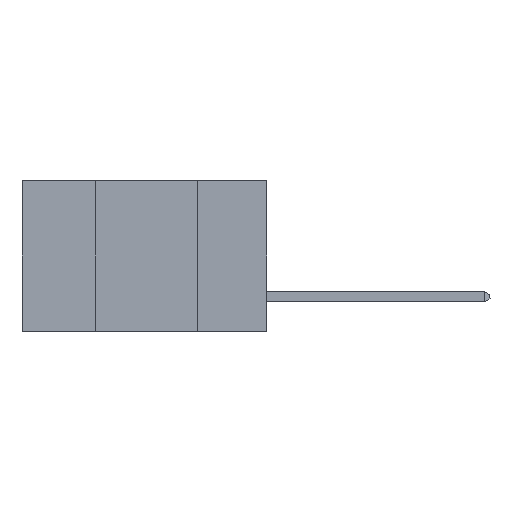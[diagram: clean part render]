
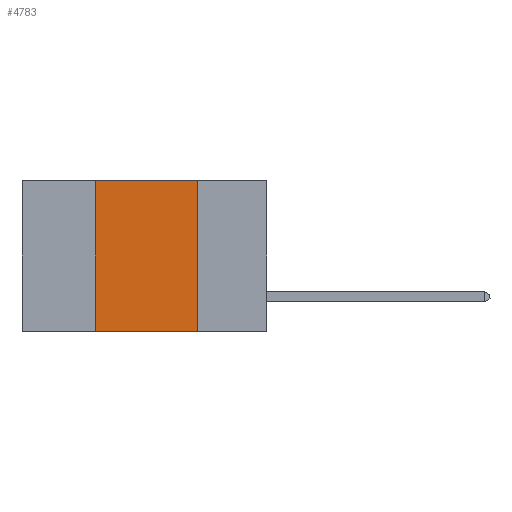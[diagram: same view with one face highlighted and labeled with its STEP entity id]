
A CAD part, left-side view. The second image highlights one B-rep face of the part: STEP entity #4783.
In plain terms, the highlighted planar face has unit normal (-1, 0, 0).
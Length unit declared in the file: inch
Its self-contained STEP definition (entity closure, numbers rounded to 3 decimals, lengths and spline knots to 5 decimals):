
#165 = EDGE_CURVE ( 'NONE', #9368, #6604, #4539, .T. ) ;
#804 = CARTESIAN_POINT ( 'NONE',  ( 0., 0.42, 0. ) ) ;
#1137 = CARTESIAN_POINT ( 'NONE',  ( 0., 0.6, 0. ) ) ;
#1305 = PLANE ( 'NONE',  #2064 ) ;
#1721 = CARTESIAN_POINT ( 'NONE',  ( 0., 0.42, -0.37 ) ) ;
#1871 = ORIENTED_EDGE ( 'NONE', *, *, #9685, .F. ) ;
#2020 = DIRECTION ( 'NONE',  ( 0., -1., 0. ) ) ;
#2064 = AXIS2_PLACEMENT_3D ( 'NONE', #1137, #6656, #10826 ) ;
#2106 = DIRECTION ( 'NONE',  ( 0., -1., 0. ) ) ;
#2413 = ORIENTED_EDGE ( 'NONE', *, *, #9881, .T. ) ;
#2480 = VERTEX_POINT ( 'NONE', #1721 ) ;
#2766 = CARTESIAN_POINT ( 'NONE',  ( 0., 0.17, -0.37 ) ) ;
#2978 = CARTESIAN_POINT ( 'NONE',  ( 0., 0.6, -0.37 ) ) ;
#3915 = VERTEX_POINT ( 'NONE', #804 ) ;
#3916 = CARTESIAN_POINT ( 'NONE',  ( 0., 0.17, 0. ) ) ;
#3965 = ORIENTED_EDGE ( 'NONE', *, *, #6851, .F. ) ;
#4436 = CARTESIAN_POINT ( 'NONE',  ( 0., 0.6, 0. ) ) ;
#4508 = LINE ( 'NONE', #5103, #11905 ) ;
#4539 = LINE ( 'NONE', #6507, #8854 ) ;
#4783 = ADVANCED_FACE ( 'NONE', ( #9858 ), #1305, .F. ) ;
#5103 = CARTESIAN_POINT ( 'NONE',  ( 0., 0.42, 0. ) ) ;
#5747 = ORIENTED_EDGE ( 'NONE', *, *, #165, .F. ) ;
#6507 = CARTESIAN_POINT ( 'NONE',  ( 0., 0.17, 0. ) ) ;
#6604 = VERTEX_POINT ( 'NONE', #2766 ) ;
#6656 = DIRECTION ( 'NONE',  ( 1., 0., 0. ) ) ;
#6683 = EDGE_LOOP ( 'NONE', ( #5747, #3965, #1871, #2413 ) ) ;
#6851 = EDGE_CURVE ( 'NONE', #3915, #9368, #10372, .T. ) ;
#8537 = VECTOR ( 'NONE', #2106, 39.37008 ) ;
#8854 = VECTOR ( 'NONE', #9235, 39.37008 ) ;
#9235 = DIRECTION ( 'NONE',  ( 0., 0., -1. ) ) ;
#9368 = VERTEX_POINT ( 'NONE', #3916 ) ;
#9685 = EDGE_CURVE ( 'NONE', #2480, #3915, #4508, .T. ) ;
#9858 = FACE_OUTER_BOUND ( 'NONE', #6683, .T. ) ;
#9881 = EDGE_CURVE ( 'NONE', #2480, #6604, #11314, .T. ) ;
#9957 = VECTOR ( 'NONE', #2020, 39.37008 ) ;
#10372 = LINE ( 'NONE', #4436, #9957 ) ;
#10826 = DIRECTION ( 'NONE',  ( 0., 0., -1. ) ) ;
#11314 = LINE ( 'NONE', #2978, #8537 ) ;
#11662 = DIRECTION ( 'NONE',  ( 0., 0., 1. ) ) ;
#11905 = VECTOR ( 'NONE', #11662, 39.37008 ) ;
